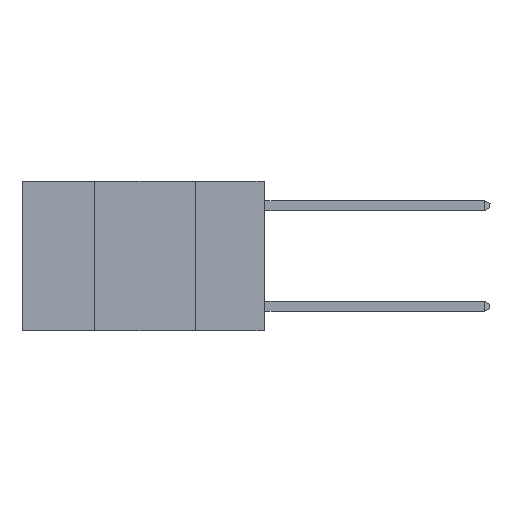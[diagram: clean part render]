
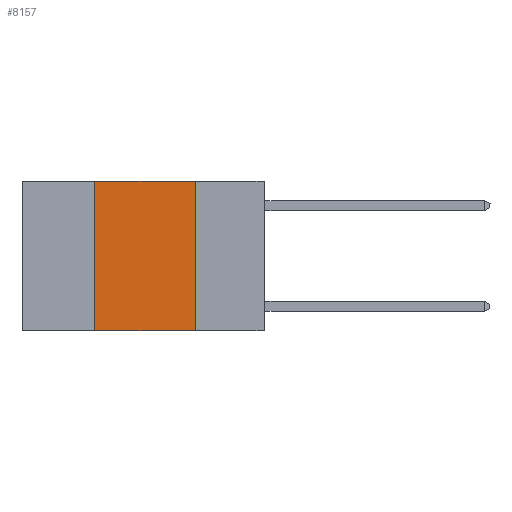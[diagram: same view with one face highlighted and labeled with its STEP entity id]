
A CAD part, left-side view. The second image highlights one B-rep face of the part: STEP entity #8157.
In plain terms, the highlighted planar face has unit normal (-1, 0, 0).
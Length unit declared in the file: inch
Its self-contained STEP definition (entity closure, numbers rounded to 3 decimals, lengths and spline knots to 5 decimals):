
#733 = CARTESIAN_POINT ( 'NONE',  ( 0., 0.6, 0. ) ) ;
#742 = VERTEX_POINT ( 'NONE', #20765 ) ;
#1319 = DIRECTION ( 'NONE',  ( 1., 0., 0. ) ) ;
#1511 = ORIENTED_EDGE ( 'NONE', *, *, #7434, .T. ) ;
#2767 = VECTOR ( 'NONE', #8767, 39.37008 ) ;
#2922 = EDGE_LOOP ( 'NONE', ( #5352, #20615, #11587, #1511 ) ) ;
#3849 = LINE ( 'NONE', #733, #4868 ) ;
#4868 = VECTOR ( 'NONE', #14286, 39.37008 ) ;
#5352 = ORIENTED_EDGE ( 'NONE', *, *, #9971, .F. ) ;
#6223 = CARTESIAN_POINT ( 'NONE',  ( 0., 0.17, -0.37 ) ) ;
#6910 = CARTESIAN_POINT ( 'NONE',  ( 0., 0.6, -0.37 ) ) ;
#6925 = EDGE_CURVE ( 'NONE', #20988, #12989, #14028, .T. ) ;
#7434 = EDGE_CURVE ( 'NONE', #20988, #16925, #15738, .T. ) ;
#7506 = VECTOR ( 'NONE', #11325, 39.37008 ) ;
#8157 = ADVANCED_FACE ( 'NONE', ( #15438 ), #12043, .F. ) ;
#8358 = AXIS2_PLACEMENT_3D ( 'NONE', #20731, #1319, #11705 ) ;
#8767 = DIRECTION ( 'NONE',  ( 0., -1., 0. ) ) ;
#9971 = EDGE_CURVE ( 'NONE', #742, #16925, #11552, .T. ) ;
#11325 = DIRECTION ( 'NONE',  ( 0., 0., -1. ) ) ;
#11552 = LINE ( 'NONE', #13330, #7506 ) ;
#11587 = ORIENTED_EDGE ( 'NONE', *, *, #6925, .F. ) ;
#11705 = DIRECTION ( 'NONE',  ( 0., 0., -1. ) ) ;
#12043 = PLANE ( 'NONE',  #8358 ) ;
#12989 = VERTEX_POINT ( 'NONE', #17664 ) ;
#13330 = CARTESIAN_POINT ( 'NONE',  ( 0., 0.17, 0. ) ) ;
#14028 = LINE ( 'NONE', #21290, #15686 ) ;
#14286 = DIRECTION ( 'NONE',  ( 0., -1., 0. ) ) ;
#15438 = FACE_OUTER_BOUND ( 'NONE', #2922, .T. ) ;
#15686 = VECTOR ( 'NONE', #17471, 39.37008 ) ;
#15738 = LINE ( 'NONE', #6910, #2767 ) ;
#16339 = EDGE_CURVE ( 'NONE', #12989, #742, #3849, .T. ) ;
#16925 = VERTEX_POINT ( 'NONE', #6223 ) ;
#17471 = DIRECTION ( 'NONE',  ( 0., 0., 1. ) ) ;
#17664 = CARTESIAN_POINT ( 'NONE',  ( 0., 0.42, 0. ) ) ;
#18741 = CARTESIAN_POINT ( 'NONE',  ( 0., 0.42, -0.37 ) ) ;
#20615 = ORIENTED_EDGE ( 'NONE', *, *, #16339, .F. ) ;
#20731 = CARTESIAN_POINT ( 'NONE',  ( 0., 0.6, 0. ) ) ;
#20765 = CARTESIAN_POINT ( 'NONE',  ( 0., 0.17, 0. ) ) ;
#20988 = VERTEX_POINT ( 'NONE', #18741 ) ;
#21290 = CARTESIAN_POINT ( 'NONE',  ( 0., 0.42, 0. ) ) ;
